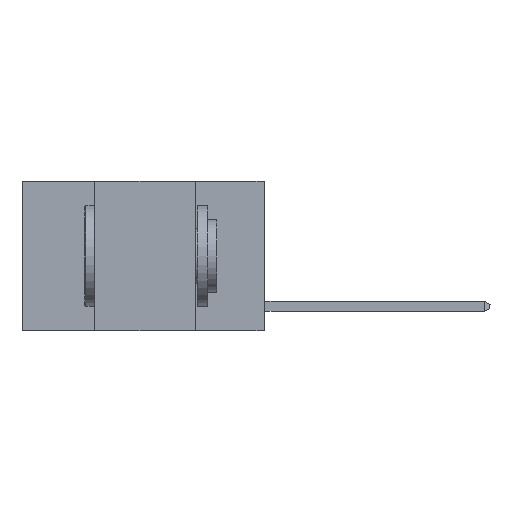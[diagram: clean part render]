
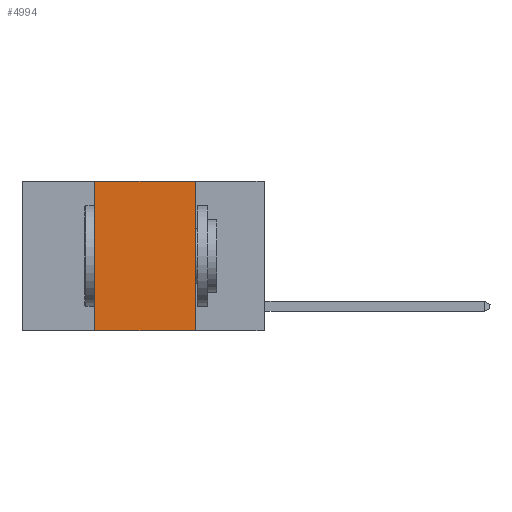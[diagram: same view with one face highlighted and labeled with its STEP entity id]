
A CAD part, left-side view. The second image highlights one B-rep face of the part: STEP entity #4994.
In plain terms, the highlighted planar face has unit normal (-1, 0, 0).
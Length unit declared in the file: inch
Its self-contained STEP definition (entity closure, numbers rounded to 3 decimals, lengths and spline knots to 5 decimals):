
#84 = DIRECTION ( 'NONE',  ( 0., 0., -1. ) ) ;
#461 = VECTOR ( 'NONE', #84, 39.37008 ) ;
#842 = CARTESIAN_POINT ( 'NONE',  ( 0., 0.6, -0.37 ) ) ;
#968 = LINE ( 'NONE', #4036, #5816 ) ;
#1129 = CARTESIAN_POINT ( 'NONE',  ( 0., 0.6, 0. ) ) ;
#1207 = VECTOR ( 'NONE', #2394, 39.37008 ) ;
#1226 = EDGE_LOOP ( 'NONE', ( #11059, #8845, #5368, #4896 ) ) ;
#1271 = DIRECTION ( 'NONE',  ( 0., 0., -1. ) ) ;
#2179 = DIRECTION ( 'NONE',  ( 0., -1., 0. ) ) ;
#2242 = PLANE ( 'NONE',  #7028 ) ;
#2394 = DIRECTION ( 'NONE',  ( 0., 0., 1. ) ) ;
#2534 = CARTESIAN_POINT ( 'NONE',  ( 0., 0.17, 0. ) ) ;
#2738 = EDGE_CURVE ( 'NONE', #3791, #7444, #8238, .T. ) ;
#2919 = CARTESIAN_POINT ( 'NONE',  ( 0., 0.42, -0.37 ) ) ;
#3021 = CARTESIAN_POINT ( 'NONE',  ( 0., 0.42, 0. ) ) ;
#3791 = VERTEX_POINT ( 'NONE', #2919 ) ;
#3830 = CARTESIAN_POINT ( 'NONE',  ( 0., 0.42, 0. ) ) ;
#4036 = CARTESIAN_POINT ( 'NONE',  ( 0., 0.6, 0. ) ) ;
#4340 = VERTEX_POINT ( 'NONE', #3830 ) ;
#4826 = FACE_OUTER_BOUND ( 'NONE', #1226, .T. ) ;
#4896 = ORIENTED_EDGE ( 'NONE', *, *, #2738, .T. ) ;
#4994 = ADVANCED_FACE ( 'NONE', ( #4826 ), #2242, .F. ) ;
#5174 = LINE ( 'NONE', #9301, #461 ) ;
#5368 = ORIENTED_EDGE ( 'NONE', *, *, #9742, .F. ) ;
#5816 = VECTOR ( 'NONE', #2179, 39.37008 ) ;
#6167 = CARTESIAN_POINT ( 'NONE',  ( 0., 0.17, -0.37 ) ) ;
#6465 = LINE ( 'NONE', #3021, #1207 ) ;
#7028 = AXIS2_PLACEMENT_3D ( 'NONE', #1129, #11319, #1271 ) ;
#7365 = VECTOR ( 'NONE', #8963, 39.37008 ) ;
#7444 = VERTEX_POINT ( 'NONE', #6167 ) ;
#7465 = VERTEX_POINT ( 'NONE', #2534 ) ;
#7529 = EDGE_CURVE ( 'NONE', #4340, #7465, #968, .T. ) ;
#8238 = LINE ( 'NONE', #842, #7365 ) ;
#8845 = ORIENTED_EDGE ( 'NONE', *, *, #7529, .F. ) ;
#8963 = DIRECTION ( 'NONE',  ( 0., -1., 0. ) ) ;
#9301 = CARTESIAN_POINT ( 'NONE',  ( 0., 0.17, 0. ) ) ;
#9742 = EDGE_CURVE ( 'NONE', #3791, #4340, #6465, .T. ) ;
#11059 = ORIENTED_EDGE ( 'NONE', *, *, #11639, .F. ) ;
#11319 = DIRECTION ( 'NONE',  ( 1., 0., 0. ) ) ;
#11639 = EDGE_CURVE ( 'NONE', #7465, #7444, #5174, .T. ) ;
